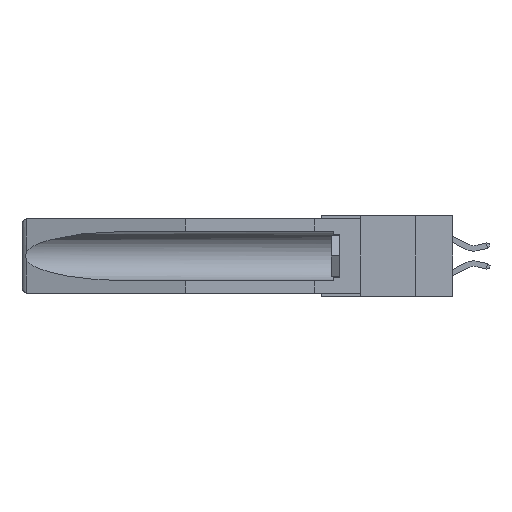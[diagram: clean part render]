
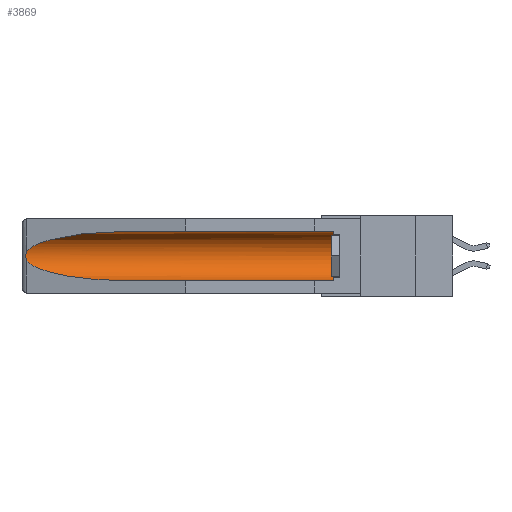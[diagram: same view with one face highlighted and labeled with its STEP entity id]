
A CAD part, left-side view. The second image highlights one B-rep face of the part: STEP entity #3869.
In plain terms, the highlighted cylindrical face has radius 2.857 mm (diameter 5.715 mm), a partial arc.
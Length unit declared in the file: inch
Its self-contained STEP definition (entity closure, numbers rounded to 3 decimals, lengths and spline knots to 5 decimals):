
#595 = EDGE_CURVE ( 'NONE', #13080, #5459, #6867, .T. ) ;
#670 = ORIENTED_EDGE ( 'NONE', *, *, #1981, .F. ) ;
#769 = CARTESIAN_POINT ( 'NONE',  ( 0.26537, 1.52718, -0.19328 ) ) ;
#838 = CARTESIAN_POINT ( 'NONE',  ( 0.26537, 1.52718, -0.19328 ) ) ;
#966 = DIRECTION ( 'NONE',  ( 0., 1., 0. ) ) ;
#1447 = CARTESIAN_POINT ( 'NONE',  ( 0.26597, 1.52961, -0.15275 ) ) ;
#1957 = CARTESIAN_POINT ( 'NONE',  ( 0.25451, 1.48313, -0.24835 ) ) ;
#1981 = EDGE_CURVE ( 'NONE', #13080, #10019, #8818, .T. ) ;
#2067 = FACE_OUTER_BOUND ( 'NONE', #16602, .T. ) ;
#2535 = VERTEX_POINT ( 'NONE', #10442 ) ;
#3023 =( BOUNDED_CURVE ( )  B_SPLINE_CURVE ( 3, ( #5262, #8992, #10563, #14661 ),
 .UNSPECIFIED., .F., .F. ) 
 B_SPLINE_CURVE_WITH_KNOTS ( ( 4, 4 ),
 ( 4.71239, 6.08839 ),
 .UNSPECIFIED. ) 
 CURVE ( )  GEOMETRIC_REPRESENTATION_ITEM ( )  RATIONAL_B_SPLINE_CURVE ( ( 1., 0.848, 0.848, 1. ) ) 
 REPRESENTATION_ITEM ( '' )  );
#3869 = ADVANCED_FACE ( 'NONE', ( #2067 ), #8538, .F. ) ;
#4052 = CARTESIAN_POINT ( 'NONE',  ( 0.155, 1.07973, -0.284 ) ) ;
#4273 = DIRECTION ( 'NONE',  ( 0., 0., 1. ) ) ;
#4296 = CARTESIAN_POINT ( 'NONE',  ( 0.26654, 1.53092, -0.15636 ) ) ;
#4362 = ORIENTED_EDGE ( 'NONE', *, *, #6553, .T. ) ;
#4850 = CARTESIAN_POINT ( 'NONE',  ( 0.155, 1.07973, -0.284 ) ) ;
#5262 = CARTESIAN_POINT ( 'NONE',  ( 0.155, 1.07973, -0.059 ) ) ;
#5459 = VERTEX_POINT ( 'NONE', #6059 ) ;
#5728 = ORIENTED_EDGE ( 'NONE', *, *, #595, .T. ) ;
#6059 = CARTESIAN_POINT ( 'NONE',  ( 0.155, 0.126, -0.059 ) ) ;
#6075 = ORIENTED_EDGE ( 'NONE', *, *, #12201, .T. ) ;
#6359 = CARTESIAN_POINT ( 'NONE',  ( 0.26537, 1.52718, -0.14972 ) ) ;
#6553 = EDGE_CURVE ( 'NONE', #5459, #2535, #12252, .T. ) ;
#6867 = CIRCLE ( 'NONE', #15254, 0.1125 ) ;
#6924 = CARTESIAN_POINT ( 'NONE',  ( 0.2673, 1.53269, -0.17917 ) ) ;
#6975 = CARTESIAN_POINT ( 'NONE',  ( 0.26537, 1.52718, -0.14972 ) ) ;
#7222 = DIRECTION ( 'NONE',  ( 0., 1., 0. ) ) ;
#7757 = DIRECTION ( 'NONE',  ( 0., 0., 1. ) ) ;
#7953 = B_SPLINE_CURVE_WITH_KNOTS ( 'NONE', 3,
 ( #6975, #1447, #4296, #16076, #16132, #12126, #6924, #8098, #10878, #13416 ),
 .UNSPECIFIED., .F., .F.,
 ( 4, 2, 2, 2, 4 ),
 ( 0., 0.00029, 0.00058, 0.00087, 0.00117 ),
 .UNSPECIFIED. ) ;
#8098 = CARTESIAN_POINT ( 'NONE',  ( 0.26655, 1.53094, -0.18657 ) ) ;
#8265 = VECTOR ( 'NONE', #7222, 39.37008 ) ;
#8376 = CARTESIAN_POINT ( 'NONE',  ( 0.155, 0.126, -0.284 ) ) ;
#8538 = CYLINDRICAL_SURFACE ( 'NONE', #16254, 0.1125 ) ;
#8818 = LINE ( 'NONE', #10512, #9022 ) ;
#8992 = CARTESIAN_POINT ( 'NONE',  ( 0.21114, 1.30732, -0.059 ) ) ;
#9022 = VECTOR ( 'NONE', #966, 39.37008 ) ;
#10019 = VERTEX_POINT ( 'NONE', #4052 ) ;
#10140 = CARTESIAN_POINT ( 'NONE',  ( 0.21114, 1.30732, -0.284 ) ) ;
#10294 = CARTESIAN_POINT ( 'NONE',  ( 0.155, -0.30754, -0.1715 ) ) ;
#10436 = EDGE_CURVE ( 'NONE', #11961, #10892, #7953, .T. ) ;
#10442 = CARTESIAN_POINT ( 'NONE',  ( 0.155, 1.07973, -0.059 ) ) ;
#10512 = CARTESIAN_POINT ( 'NONE',  ( 0.155, -0.30754, -0.284 ) ) ;
#10563 = CARTESIAN_POINT ( 'NONE',  ( 0.25451, 1.48313, -0.09465 ) ) ;
#10878 = CARTESIAN_POINT ( 'NONE',  ( 0.26597, 1.5296, -0.19026 ) ) ;
#10892 = VERTEX_POINT ( 'NONE', #838 ) ;
#11950 = EDGE_CURVE ( 'NONE', #2535, #11961, #3023, .T. ) ;
#11961 = VERTEX_POINT ( 'NONE', #6359 ) ;
#12126 = CARTESIAN_POINT ( 'NONE',  ( 0.2675, 1.53308, -0.17534 ) ) ;
#12201 = EDGE_CURVE ( 'NONE', #10892, #10019, #15727, .T. ) ;
#12252 = LINE ( 'NONE', #12378, #8265 ) ;
#12281 = CARTESIAN_POINT ( 'NONE',  ( 0.155, 0.126, -0.1715 ) ) ;
#12378 = CARTESIAN_POINT ( 'NONE',  ( 0.155, -0.30754, -0.059 ) ) ;
#13080 = VERTEX_POINT ( 'NONE', #8376 ) ;
#13416 = CARTESIAN_POINT ( 'NONE',  ( 0.26537, 1.52718, -0.19328 ) ) ;
#13763 = ORIENTED_EDGE ( 'NONE', *, *, #11950, .T. ) ;
#14661 = CARTESIAN_POINT ( 'NONE',  ( 0.26537, 1.52718, -0.14972 ) ) ;
#15148 = ORIENTED_EDGE ( 'NONE', *, *, #10436, .T. ) ;
#15254 = AXIS2_PLACEMENT_3D ( 'NONE', #12281, #16291, #4273 ) ;
#15727 =( BOUNDED_CURVE ( )  B_SPLINE_CURVE ( 3, ( #769, #1957, #10140, #4850 ),
 .UNSPECIFIED., .F., .T. ) 
 B_SPLINE_CURVE_WITH_KNOTS ( ( 4, 4 ),
 ( 0.1948, 1.5708 ),
 .UNSPECIFIED. ) 
 CURVE ( )  GEOMETRIC_REPRESENTATION_ITEM ( )  RATIONAL_B_SPLINE_CURVE ( ( 1., 0.848, 0.848, 1. ) ) 
 REPRESENTATION_ITEM ( '' )  );
#16076 = CARTESIAN_POINT ( 'NONE',  ( 0.2673, 1.5327, -0.16383 ) ) ;
#16132 = CARTESIAN_POINT ( 'NONE',  ( 0.2675, 1.53308, -0.16763 ) ) ;
#16254 = AXIS2_PLACEMENT_3D ( 'NONE', #10294, #17110, #7757 ) ;
#16291 = DIRECTION ( 'NONE',  ( 0., -1., 0. ) ) ;
#16602 = EDGE_LOOP ( 'NONE', ( #13763, #15148, #6075, #670, #5728, #4362 ) ) ;
#17110 = DIRECTION ( 'NONE',  ( 0., 1., 0. ) ) ;
